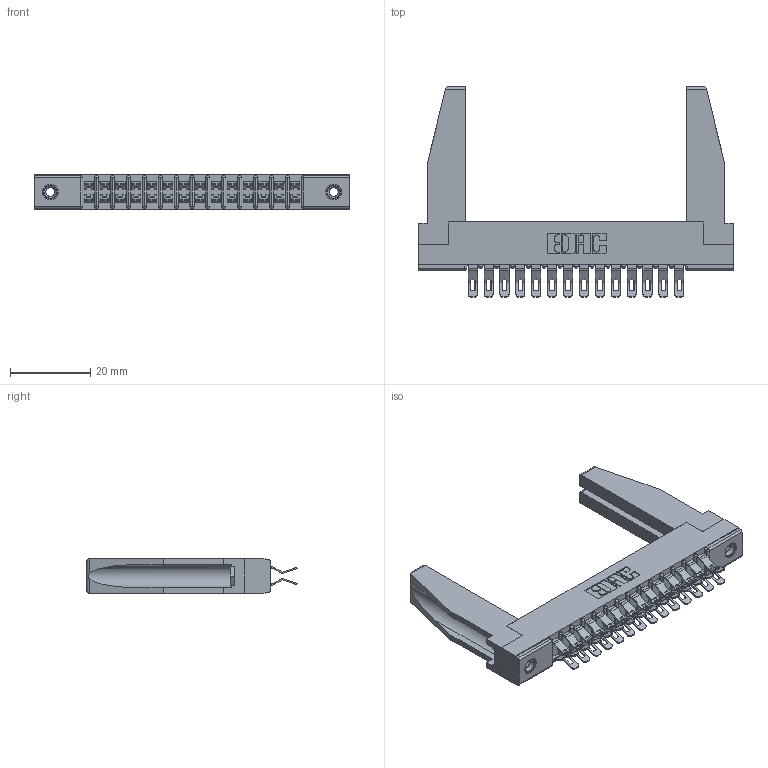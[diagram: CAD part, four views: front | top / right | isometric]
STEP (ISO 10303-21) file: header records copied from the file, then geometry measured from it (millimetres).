
FILE_DESCRIPTION (( 'STEP AP203' ), '1' );
FILE_NAME ('307-028-455-278.STEP', '2020-09-29T08:17:28', ( '' ), ( '' ), 'SwSTEP 2.0', 'SolidWorks 2020', '' );
FILE_SCHEMA (( 'CONFIG_CONTROL_DESIGN' ));
Length unit declared in the file: inch
Products named in the file (5): 345-250-001_345-250-001-102; 307-220-078; 307-290-001_555; 307-028-455-278; 307 Part_.156 Dia Mounting Holes
Assembly tree (33 placements, depth 2):
  307-028-455-278
    307 Part_.156 Dia Mounting Holes
    307-290-001_555  x28
    307-220-078  x2
    345-250-001_345-250-001-102  x2
Bounding box: 78.49 x 52.45 x 8.71 mm (x, y, z)
Volume: 9211.5 mm3; surface area: 13084.1 mm2
Topology: 33 solids, 33 shells, 1971 faces, 5721 edges, 3726 vertices
Faces by surface type: plane 1106, cylinder 819, sphere 30, cone 12, torus 4
Entity records: 18878 total; most frequent: CARTESIAN_POINT 3112, ORIENTED_EDGE 3042, DIRECTION 3021, EDGE_CURVE 1521, VECTOR 1147, LINE 1147, VERTEX_POINT 986, AXIS2_PLACEMENT_3D 937
